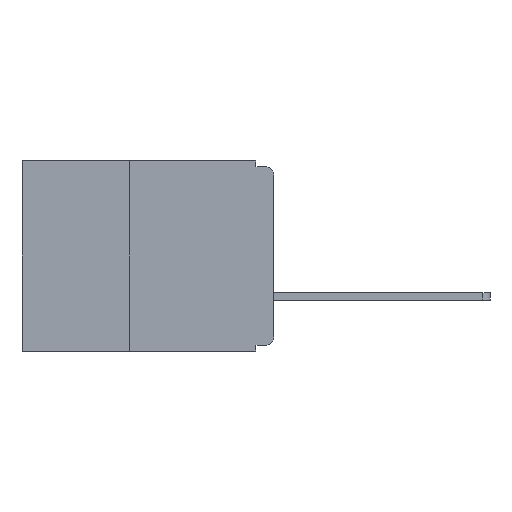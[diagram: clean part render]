
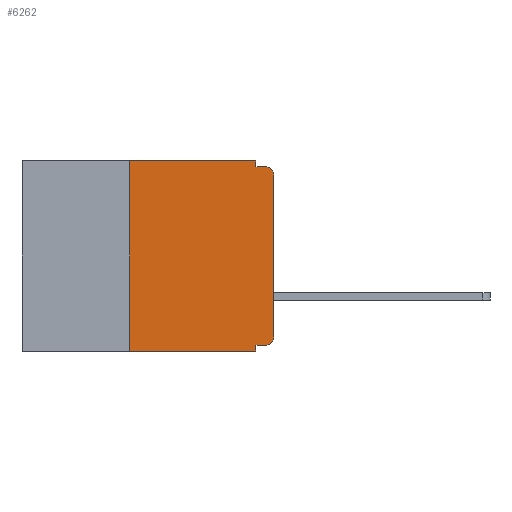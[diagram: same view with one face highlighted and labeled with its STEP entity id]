
A CAD part, left-side view. The second image highlights one B-rep face of the part: STEP entity #6262.
In plain terms, the highlighted planar face has unit normal (-1, 0, 0).
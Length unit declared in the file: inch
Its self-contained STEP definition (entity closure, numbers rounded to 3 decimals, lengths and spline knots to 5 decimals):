
#10 = VERTEX_POINT ( 'NONE', #21434 ) ;
#59 = CARTESIAN_POINT ( 'NONE',  ( 0., 0.25, -0.33 ) ) ;
#180 = FACE_OUTER_BOUND ( 'NONE', #21307, .T. ) ;
#989 = CARTESIAN_POINT ( 'NONE',  ( 0., 0.437, 0. ) ) ;
#1233 = VECTOR ( 'NONE', #21003, 39.37008 ) ;
#1655 = ORIENTED_EDGE ( 'NONE', *, *, #22637, .F. ) ;
#2728 = VECTOR ( 'NONE', #25247, 39.37008 ) ;
#2917 = EDGE_CURVE ( 'NONE', #3626, #3599, #14202, .T. ) ;
#2952 = DIRECTION ( 'NONE',  ( 1., 0., 0. ) ) ;
#3568 = CARTESIAN_POINT ( 'NONE',  ( 0., 0., -0.01 ) ) ;
#3599 = VERTEX_POINT ( 'NONE', #25300 ) ;
#3600 = EDGE_CURVE ( 'NONE', #16827, #3626, #7966, .T. ) ;
#3626 = VERTEX_POINT ( 'NONE', #25166 ) ;
#3650 = DIRECTION ( 'NONE',  ( 0., -1., 0. ) ) ;
#3837 = VERTEX_POINT ( 'NONE', #20694 ) ;
#3870 = LINE ( 'NONE', #21600, #7867 ) ;
#5611 = CARTESIAN_POINT ( 'NONE',  ( 0., 0., 0. ) ) ;
#5750 = ORIENTED_EDGE ( 'NONE', *, *, #6948, .F. ) ;
#6151 = EDGE_CURVE ( 'NONE', #15823, #12555, #17788, .T. ) ;
#6262 = ADVANCED_FACE ( 'NONE', ( #180 ), #24488, .F. ) ;
#6351 = ORIENTED_EDGE ( 'NONE', *, *, #6151, .F. ) ;
#6547 = EDGE_CURVE ( 'NONE', #3599, #21842, #3870, .T. ) ;
#6948 = EDGE_CURVE ( 'NONE', #12555, #16945, #8446, .T. ) ;
#7201 = ORIENTED_EDGE ( 'NONE', *, *, #6547, .F. ) ;
#7436 = VECTOR ( 'NONE', #7586, 39.37008 ) ;
#7586 = DIRECTION ( 'NONE',  ( 0., 0., 1. ) ) ;
#7611 = VERTEX_POINT ( 'NONE', #21120 ) ;
#7867 = VECTOR ( 'NONE', #13746, 39.37008 ) ;
#7966 = LINE ( 'NONE', #59, #2728 ) ;
#8446 = LINE ( 'NONE', #13280, #25320 ) ;
#8537 = DIRECTION ( 'NONE',  ( 0., 1., 0. ) ) ;
#8914 = VECTOR ( 'NONE', #14868, 39.37008 ) ;
#9084 = CARTESIAN_POINT ( 'NONE',  ( 0., 0.031, -0.01 ) ) ;
#9297 = ORIENTED_EDGE ( 'NONE', *, *, #23204, .T. ) ;
#9716 = ORIENTED_EDGE ( 'NONE', *, *, #24824, .T. ) ;
#11341 = DIRECTION ( 'NONE',  ( -1., 0., 0. ) ) ;
#11421 = VECTOR ( 'NONE', #3650, 39.37008 ) ;
#11508 = CARTESIAN_POINT ( 'NONE',  ( 0., 0.015, -0.025 ) ) ;
#12063 = CIRCLE ( 'NONE', #18967, 0.015 ) ;
#12341 = CARTESIAN_POINT ( 'NONE',  ( 0., 0.015, -0.32 ) ) ;
#12514 = EDGE_CURVE ( 'NONE', #15823, #7611, #15049, .T. ) ;
#12555 = VERTEX_POINT ( 'NONE', #13451 ) ;
#12686 = LINE ( 'NONE', #3568, #11421 ) ;
#13161 = VECTOR ( 'NONE', #8537, 39.37008 ) ;
#13280 = CARTESIAN_POINT ( 'NONE',  ( 0., 0.031, -0.33 ) ) ;
#13451 = CARTESIAN_POINT ( 'NONE',  ( 0., 0.031, -0.32 ) ) ;
#13537 = DIRECTION ( 'NONE',  ( 0., 0., -1. ) ) ;
#13746 = DIRECTION ( 'NONE',  ( 0., 0., -1. ) ) ;
#14202 = LINE ( 'NONE', #20804, #8914 ) ;
#14470 = AXIS2_PLACEMENT_3D ( 'NONE', #23104, #11341, #25040 ) ;
#14868 = DIRECTION ( 'NONE',  ( 0., -1., 0. ) ) ;
#15049 = CIRCLE ( 'NONE', #14470, 0.015 ) ;
#15823 = VERTEX_POINT ( 'NONE', #12341 ) ;
#16643 = EDGE_CURVE ( 'NONE', #3837, #10, #12063, .T. ) ;
#16710 = CARTESIAN_POINT ( 'NONE',  ( 0., 0.25, -0.33 ) ) ;
#16757 = DIRECTION ( 'NONE',  ( 0., 0., -1. ) ) ;
#16794 = ORIENTED_EDGE ( 'NONE', *, *, #2917, .F. ) ;
#16827 = VERTEX_POINT ( 'NONE', #16710 ) ;
#16945 = VERTEX_POINT ( 'NONE', #19344 ) ;
#17583 = LINE ( 'NONE', #19042, #1233 ) ;
#17788 = LINE ( 'NONE', #18377, #13161 ) ;
#18377 = CARTESIAN_POINT ( 'NONE',  ( 0., 0., -0.32 ) ) ;
#18383 = AXIS2_PLACEMENT_3D ( 'NONE', #989, #2952, #16757 ) ;
#18677 = ORIENTED_EDGE ( 'NONE', *, *, #12514, .T. ) ;
#18967 = AXIS2_PLACEMENT_3D ( 'NONE', #11508, #25199, #13537 ) ;
#19042 = CARTESIAN_POINT ( 'NONE',  ( 0., 0.437, -0.33 ) ) ;
#19344 = CARTESIAN_POINT ( 'NONE',  ( 0., 0.031, -0.33 ) ) ;
#19492 = ORIENTED_EDGE ( 'NONE', *, *, #16643, .T. ) ;
#20694 = CARTESIAN_POINT ( 'NONE',  ( 0., 0., -0.025 ) ) ;
#20804 = CARTESIAN_POINT ( 'NONE',  ( 0., 0.437, 0. ) ) ;
#21003 = DIRECTION ( 'NONE',  ( 0., -1., 0. ) ) ;
#21069 = ORIENTED_EDGE ( 'NONE', *, *, #3600, .F. ) ;
#21120 = CARTESIAN_POINT ( 'NONE',  ( 0., 0., -0.305 ) ) ;
#21307 = EDGE_LOOP ( 'NONE', ( #9297, #19492, #1655, #7201, #16794, #21069, #9716, #5750, #6351, #18677 ) ) ;
#21434 = CARTESIAN_POINT ( 'NONE',  ( 0., 0.015, -0.01 ) ) ;
#21600 = CARTESIAN_POINT ( 'NONE',  ( 0., 0.031, 0. ) ) ;
#21842 = VERTEX_POINT ( 'NONE', #9084 ) ;
#22637 = EDGE_CURVE ( 'NONE', #21842, #10, #12686, .T. ) ;
#23103 = LINE ( 'NONE', #5611, #7436 ) ;
#23104 = CARTESIAN_POINT ( 'NONE',  ( 0., 0.015, -0.305 ) ) ;
#23204 = EDGE_CURVE ( 'NONE', #7611, #3837, #23103, .T. ) ;
#24488 = PLANE ( 'NONE',  #18383 ) ;
#24824 = EDGE_CURVE ( 'NONE', #16827, #16945, #17583, .T. ) ;
#24958 = DIRECTION ( 'NONE',  ( 0., 0., -1. ) ) ;
#25040 = DIRECTION ( 'NONE',  ( 0., 0., -1. ) ) ;
#25166 = CARTESIAN_POINT ( 'NONE',  ( 0., 0.25, 0. ) ) ;
#25199 = DIRECTION ( 'NONE',  ( -1., 0., 0. ) ) ;
#25247 = DIRECTION ( 'NONE',  ( 0., 0., 1. ) ) ;
#25300 = CARTESIAN_POINT ( 'NONE',  ( 0., 0.031, 0. ) ) ;
#25320 = VECTOR ( 'NONE', #24958, 39.37008 ) ;
